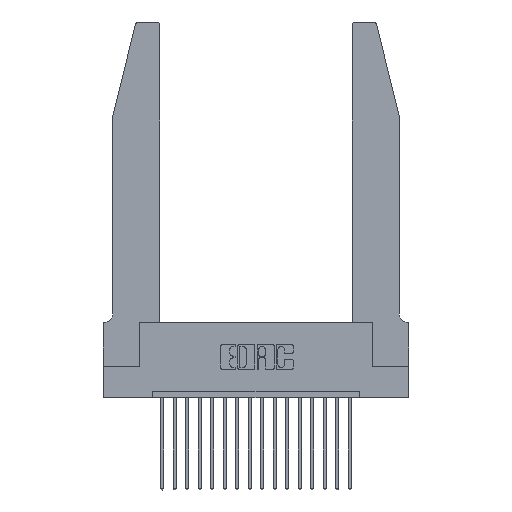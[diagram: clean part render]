
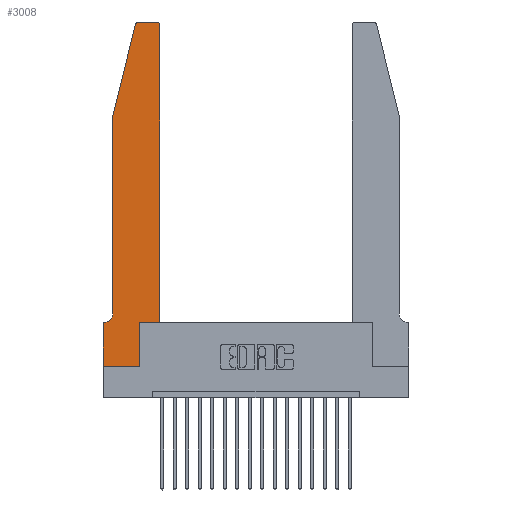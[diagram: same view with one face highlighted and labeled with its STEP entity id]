
A CAD part, top view. The second image highlights one B-rep face of the part: STEP entity #3008.
In plain terms, the highlighted planar face has unit normal (0, 0, 1).
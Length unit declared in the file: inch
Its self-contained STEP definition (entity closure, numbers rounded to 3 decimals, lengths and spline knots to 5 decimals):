
#224 = CARTESIAN_POINT ( 'NONE',  ( 0.2605, 2.75, 0.37 ) ) ;
#229 = VERTEX_POINT ( 'NONE', #14365 ) ;
#352 = LINE ( 'NONE', #6366, #12900 ) ;
#673 = ORIENTED_EDGE ( 'NONE', *, *, #5986, .T. ) ;
#811 = ORIENTED_EDGE ( 'NONE', *, *, #1816, .T. ) ;
#813 = ORIENTED_EDGE ( 'NONE', *, *, #19829, .T. ) ;
#1648 = ORIENTED_EDGE ( 'NONE', *, *, #19916, .T. ) ;
#1816 = EDGE_CURVE ( 'NONE', #4586, #3020, #14758, .T. ) ;
#1884 = DIRECTION ( 'NONE',  ( 1., 0., 0. ) ) ;
#1907 = CARTESIAN_POINT ( 'NONE',  ( 0.0755, 2., 0.37 ) ) ;
#1937 = FACE_OUTER_BOUND ( 'NONE', #7357, .T. ) ;
#1946 = ORIENTED_EDGE ( 'NONE', *, *, #13166, .T. ) ;
#2868 = CARTESIAN_POINT ( 'NONE',  ( 0.0755, 0.35, 0.37 ) ) ;
#3008 = ADVANCED_FACE ( 'NONE', ( #1937 ), #10486, .T. ) ;
#3020 = VERTEX_POINT ( 'NONE', #5672 ) ;
#3286 = DIRECTION ( 'NONE',  ( -1., 0., 0. ) ) ;
#3711 = VERTEX_POINT ( 'NONE', #18033 ) ;
#3891 = EDGE_CURVE ( 'NONE', #3020, #229, #9101, .T. ) ;
#4027 = DIRECTION ( 'NONE',  ( 1., 0., 0. ) ) ;
#4248 = VERTEX_POINT ( 'NONE', #9122 ) ;
#4440 = VECTOR ( 'NONE', #4837, 39.37008 ) ;
#4547 = LINE ( 'NONE', #1907, #13393 ) ;
#4586 = VERTEX_POINT ( 'NONE', #12432 ) ;
#4724 = DIRECTION ( 'NONE',  ( 0., 0., -1. ) ) ;
#4786 = ORIENTED_EDGE ( 'NONE', *, *, #9595, .T. ) ;
#4837 = DIRECTION ( 'NONE',  ( 1., 0., 0. ) ) ;
#5033 = DIRECTION ( 'NONE',  ( 0., 1., 0. ) ) ;
#5092 = VECTOR ( 'NONE', #7713, 39.37008 ) ;
#5672 = CARTESIAN_POINT ( 'NONE',  ( 0.2865, 0.35, 0.37 ) ) ;
#5776 = VECTOR ( 'NONE', #3286, 39.37008 ) ;
#5942 = DIRECTION ( 'NONE',  ( 1., 0., 0. ) ) ;
#5986 = EDGE_CURVE ( 'NONE', #6517, #13084, #18347, .T. ) ;
#6366 = CARTESIAN_POINT ( 'NONE',  ( 0.4505, 0.35, 0.37 ) ) ;
#6406 = VECTOR ( 'NONE', #5033, 39.37008 ) ;
#6442 = CIRCLE ( 'NONE', #18691, 0.03 ) ;
#6517 = VERTEX_POINT ( 'NONE', #6541 ) ;
#6541 = CARTESIAN_POINT ( 'NONE',  ( 0., 0.35, 0.37 ) ) ;
#6597 = CARTESIAN_POINT ( 'NONE',  ( 0.4505, 2.72, 0.37 ) ) ;
#7073 = EDGE_CURVE ( 'NONE', #4248, #12677, #14661, .T. ) ;
#7357 = EDGE_LOOP ( 'NONE', ( #16976, #4786, #15217, #10733, #18573, #813, #673, #19296, #811, #14201, #1648, #1946 ) ) ;
#7368 = AXIS2_PLACEMENT_3D ( 'NONE', #11400, #4724, #8142 ) ;
#7713 = DIRECTION ( 'NONE',  ( 1., 0., 0. ) ) ;
#7894 = EDGE_CURVE ( 'NONE', #14467, #9334, #4547, .T. ) ;
#7988 = CARTESIAN_POINT ( 'NONE',  ( 0.4505, 0.35, 0.37 ) ) ;
#8114 = DIRECTION ( 'NONE',  ( 0., 0., 1. ) ) ;
#8142 = DIRECTION ( 'NONE',  ( -1., 0., 0. ) ) ;
#8306 = CARTESIAN_POINT ( 'NONE',  ( 0., 0., 0.37 ) ) ;
#8973 = VECTOR ( 'NONE', #11257, 39.37008 ) ;
#9101 = LINE ( 'NONE', #7988, #4440 ) ;
#9122 = CARTESIAN_POINT ( 'NONE',  ( 0.0755, 0.42, 0.37 ) ) ;
#9334 = VERTEX_POINT ( 'NONE', #19997 ) ;
#9474 = EDGE_CURVE ( 'NONE', #9334, #4248, #14802, .T. ) ;
#9569 = CARTESIAN_POINT ( 'NONE',  ( 0., 0., 0.37 ) ) ;
#9595 = EDGE_CURVE ( 'NONE', #3711, #14467, #6442, .T. ) ;
#9835 = CARTESIAN_POINT ( 'NONE',  ( 0.2865, 0.35, 0.37 ) ) ;
#9914 = DIRECTION ( 'NONE',  ( 0., -1., 0. ) ) ;
#10486 = PLANE ( 'NONE',  #15419 ) ;
#10513 = VECTOR ( 'NONE', #9914, 39.37008 ) ;
#10721 = EDGE_CURVE ( 'NONE', #15294, #3711, #12657, .T. ) ;
#10733 = ORIENTED_EDGE ( 'NONE', *, *, #9474, .T. ) ;
#10977 = DIRECTION ( 'NONE',  ( 0., 1., 0. ) ) ;
#11257 = DIRECTION ( 'NONE',  ( -1., 0., 0. ) ) ;
#11400 = CARTESIAN_POINT ( 'NONE',  ( 0.0055, 0.42, 0.37 ) ) ;
#11486 = LINE ( 'NONE', #18601, #5092 ) ;
#11856 = CARTESIAN_POINT ( 'NONE',  ( 0.284, 2.72, 0.37 ) ) ;
#12432 = CARTESIAN_POINT ( 'NONE',  ( 0.2865, 0., 0.37 ) ) ;
#12657 = LINE ( 'NONE', #224, #8973 ) ;
#12677 = VERTEX_POINT ( 'NONE', #14999 ) ;
#12900 = VECTOR ( 'NONE', #10977, 39.37008 ) ;
#13084 = VERTEX_POINT ( 'NONE', #9569 ) ;
#13166 = EDGE_CURVE ( 'NONE', #19376, #15294, #17460, .T. ) ;
#13393 = VECTOR ( 'NONE', #19187, 39.37008 ) ;
#13413 = DIRECTION ( 'NONE',  ( 0., 0., 1. ) ) ;
#14201 = ORIENTED_EDGE ( 'NONE', *, *, #3891, .T. ) ;
#14365 = CARTESIAN_POINT ( 'NONE',  ( 0.4505, 0.35, 0.37 ) ) ;
#14467 = VERTEX_POINT ( 'NONE', #20053 ) ;
#14661 = CIRCLE ( 'NONE', #7368, 0.07 ) ;
#14758 = LINE ( 'NONE', #9835, #6406 ) ;
#14802 = LINE ( 'NONE', #16292, #19902 ) ;
#14999 = CARTESIAN_POINT ( 'NONE',  ( 0.0055, 0.35, 0.37 ) ) ;
#15027 = CARTESIAN_POINT ( 'NONE',  ( 0.4205, 2.75, 0.37 ) ) ;
#15217 = ORIENTED_EDGE ( 'NONE', *, *, #7894, .T. ) ;
#15294 = VERTEX_POINT ( 'NONE', #15027 ) ;
#15338 = DIRECTION ( 'NONE',  ( 0., 0., 1. ) ) ;
#15419 = AXIS2_PLACEMENT_3D ( 'NONE', #20038, #15338, #5942 ) ;
#16195 = EDGE_CURVE ( 'NONE', #13084, #4586, #11486, .T. ) ;
#16292 = CARTESIAN_POINT ( 'NONE',  ( 0.0755, 2., 0.37 ) ) ;
#16976 = ORIENTED_EDGE ( 'NONE', *, *, #10721, .T. ) ;
#17460 = CIRCLE ( 'NONE', #19276, 0.03 ) ;
#18033 = CARTESIAN_POINT ( 'NONE',  ( 0.284, 2.75, 0.37 ) ) ;
#18347 = LINE ( 'NONE', #8306, #10513 ) ;
#18573 = ORIENTED_EDGE ( 'NONE', *, *, #7073, .T. ) ;
#18601 = CARTESIAN_POINT ( 'NONE',  ( 0., 0., 0.37 ) ) ;
#18691 = AXIS2_PLACEMENT_3D ( 'NONE', #11856, #13413, #4027 ) ;
#19156 = CARTESIAN_POINT ( 'NONE',  ( 0.4205, 2.72, 0.37 ) ) ;
#19187 = DIRECTION ( 'NONE',  ( -0.239, -0.971, 0. ) ) ;
#19276 = AXIS2_PLACEMENT_3D ( 'NONE', #19156, #8114, #1884 ) ;
#19296 = ORIENTED_EDGE ( 'NONE', *, *, #16195, .T. ) ;
#19376 = VERTEX_POINT ( 'NONE', #6597 ) ;
#19562 = DIRECTION ( 'NONE',  ( 0., -1., 0. ) ) ;
#19829 = EDGE_CURVE ( 'NONE', #12677, #6517, #20245, .T. ) ;
#19902 = VECTOR ( 'NONE', #19562, 39.37008 ) ;
#19916 = EDGE_CURVE ( 'NONE', #229, #19376, #352, .T. ) ;
#19997 = CARTESIAN_POINT ( 'NONE',  ( 0.0755, 2., 0.37 ) ) ;
#20038 = CARTESIAN_POINT ( 'NONE',  ( 0., 0.35, 0.37 ) ) ;
#20053 = CARTESIAN_POINT ( 'NONE',  ( 0.25487, 2.72718, 0.37 ) ) ;
#20245 = LINE ( 'NONE', #2868, #5776 ) ;
